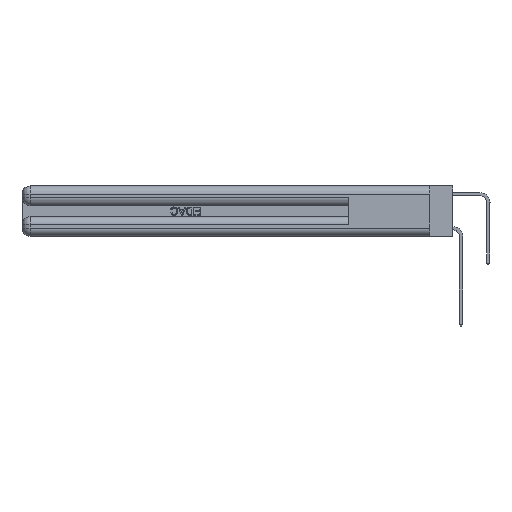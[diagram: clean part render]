
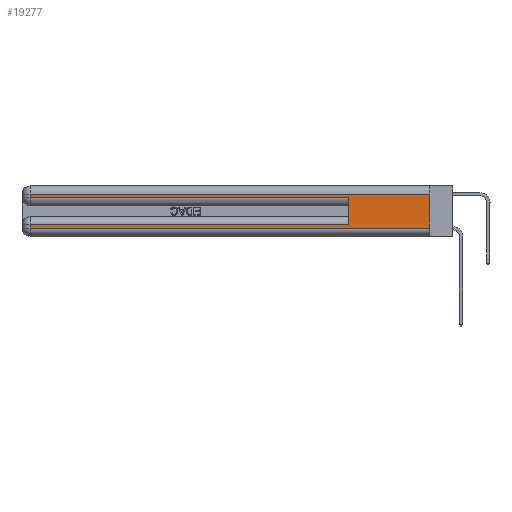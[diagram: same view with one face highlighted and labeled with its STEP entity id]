
A CAD part, left-side view. The second image highlights one B-rep face of the part: STEP entity #19277.
In plain terms, the highlighted planar face has unit normal (-1, 0, 0).
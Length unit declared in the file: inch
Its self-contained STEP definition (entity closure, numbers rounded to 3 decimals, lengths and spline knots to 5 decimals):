
#185 = EDGE_CURVE ( 'NONE', #23999, #32784, #4669, .T. ) ;
#1197 = ORIENTED_EDGE ( 'NONE', *, *, #23234, .T. ) ;
#1333 = LINE ( 'NONE', #13175, #16785 ) ;
#1801 = CARTESIAN_POINT ( 'NONE',  ( 0., 0., 0.285 ) ) ;
#2776 = LINE ( 'NONE', #8862, #16565 ) ;
#3019 = EDGE_CURVE ( 'NONE', #9516, #22471, #5544, .T. ) ;
#3367 = CARTESIAN_POINT ( 'NONE',  ( 0., 0., 0.06 ) ) ;
#3740 = VECTOR ( 'NONE', #22728, 39.37008 ) ;
#4143 = EDGE_CURVE ( 'NONE', #22471, #27634, #33402, .T. ) ;
#4669 = LINE ( 'NONE', #23271, #12000 ) ;
#5544 = LINE ( 'NONE', #26177, #9478 ) ;
#8059 = CARTESIAN_POINT ( 'NONE',  ( 0., 0.6, 0.085 ) ) ;
#8313 = FACE_OUTER_BOUND ( 'NONE', #9127, .T. ) ;
#8862 = CARTESIAN_POINT ( 'NONE',  ( 0., 0., 0.085 ) ) ;
#9127 = EDGE_LOOP ( 'NONE', ( #34541, #1197, #16146, #9316, #35364, #15912, #23691, #17499 ) ) ;
#9316 = ORIENTED_EDGE ( 'NONE', *, *, #29828, .T. ) ;
#9457 = DIRECTION ( 'NONE',  ( 0., 0., 1. ) ) ;
#9478 = VECTOR ( 'NONE', #12600, 39.37008 ) ;
#9516 = VERTEX_POINT ( 'NONE', #20438 ) ;
#10835 = CARTESIAN_POINT ( 'NONE',  ( 0., 0., 0.06 ) ) ;
#12000 = VECTOR ( 'NONE', #20501, 39.37008 ) ;
#12192 = EDGE_CURVE ( 'NONE', #26528, #27634, #22303, .T. ) ;
#12600 = DIRECTION ( 'NONE',  ( 0., 0., -1. ) ) ;
#12623 = DIRECTION ( 'NONE',  ( 0., -1., 0. ) ) ;
#13175 = CARTESIAN_POINT ( 'NONE',  ( 0., 0., 0.31 ) ) ;
#13991 = CARTESIAN_POINT ( 'NONE',  ( 0., 2.94, 0.31 ) ) ;
#14496 = EDGE_CURVE ( 'NONE', #23767, #9516, #2776, .T. ) ;
#14936 = DIRECTION ( 'NONE',  ( 0., 0., -1. ) ) ;
#15912 = ORIENTED_EDGE ( 'NONE', *, *, #14496, .T. ) ;
#16146 = ORIENTED_EDGE ( 'NONE', *, *, #185, .T. ) ;
#16565 = VECTOR ( 'NONE', #28197, 39.37008 ) ;
#16785 = VECTOR ( 'NONE', #27009, 39.37008 ) ;
#17499 = ORIENTED_EDGE ( 'NONE', *, *, #4143, .T. ) ;
#17822 = DIRECTION ( 'NONE',  ( 1., 0., 0. ) ) ;
#18838 = VECTOR ( 'NONE', #23812, 39.37008 ) ;
#19277 = ADVANCED_FACE ( 'NONE', ( #8313 ), #26211, .F. ) ;
#19828 = CARTESIAN_POINT ( 'NONE',  ( 0., 0., 0.31 ) ) ;
#20438 = CARTESIAN_POINT ( 'NONE',  ( 0., 2.94, 0.085 ) ) ;
#20501 = DIRECTION ( 'NONE',  ( 0., 0., -1. ) ) ;
#22303 = LINE ( 'NONE', #26461, #18838 ) ;
#22359 = VERTEX_POINT ( 'NONE', #24821 ) ;
#22471 = VERTEX_POINT ( 'NONE', #34094 ) ;
#22728 = DIRECTION ( 'NONE',  ( 0., -1., 0. ) ) ;
#23234 = EDGE_CURVE ( 'NONE', #26528, #23999, #1333, .T. ) ;
#23271 = CARTESIAN_POINT ( 'NONE',  ( 0., 2.94, 0.37 ) ) ;
#23691 = ORIENTED_EDGE ( 'NONE', *, *, #3019, .T. ) ;
#23767 = VERTEX_POINT ( 'NONE', #8059 ) ;
#23812 = DIRECTION ( 'NONE',  ( 0., 0., -1. ) ) ;
#23999 = VERTEX_POINT ( 'NONE', #13991 ) ;
#24821 = CARTESIAN_POINT ( 'NONE',  ( 0., 0.6, 0.285 ) ) ;
#25389 = AXIS2_PLACEMENT_3D ( 'NONE', #34271, #17822, #14936 ) ;
#25885 = CARTESIAN_POINT ( 'NONE',  ( 0., 0.6, 0.145 ) ) ;
#26177 = CARTESIAN_POINT ( 'NONE',  ( 0., 2.94, 0.37 ) ) ;
#26211 = PLANE ( 'NONE',  #25389 ) ;
#26461 = CARTESIAN_POINT ( 'NONE',  ( 0., 0., 0.37 ) ) ;
#26528 = VERTEX_POINT ( 'NONE', #19828 ) ;
#27009 = DIRECTION ( 'NONE',  ( 0., 1., 0. ) ) ;
#27634 = VERTEX_POINT ( 'NONE', #10835 ) ;
#27678 = VECTOR ( 'NONE', #12623, 39.37008 ) ;
#28197 = DIRECTION ( 'NONE',  ( 0., 1., 0. ) ) ;
#28417 = EDGE_CURVE ( 'NONE', #23767, #22359, #30663, .T. ) ;
#28775 = CARTESIAN_POINT ( 'NONE',  ( 0., 2.94, 0.285 ) ) ;
#29828 = EDGE_CURVE ( 'NONE', #32784, #22359, #30677, .T. ) ;
#30663 = LINE ( 'NONE', #25885, #33259 ) ;
#30677 = LINE ( 'NONE', #1801, #27678 ) ;
#32784 = VERTEX_POINT ( 'NONE', #28775 ) ;
#33259 = VECTOR ( 'NONE', #9457, 39.37008 ) ;
#33402 = LINE ( 'NONE', #3367, #3740 ) ;
#34094 = CARTESIAN_POINT ( 'NONE',  ( 0., 2.94, 0.06 ) ) ;
#34271 = CARTESIAN_POINT ( 'NONE',  ( 0., 0., 0.37 ) ) ;
#34541 = ORIENTED_EDGE ( 'NONE', *, *, #12192, .F. ) ;
#35364 = ORIENTED_EDGE ( 'NONE', *, *, #28417, .F. ) ;
